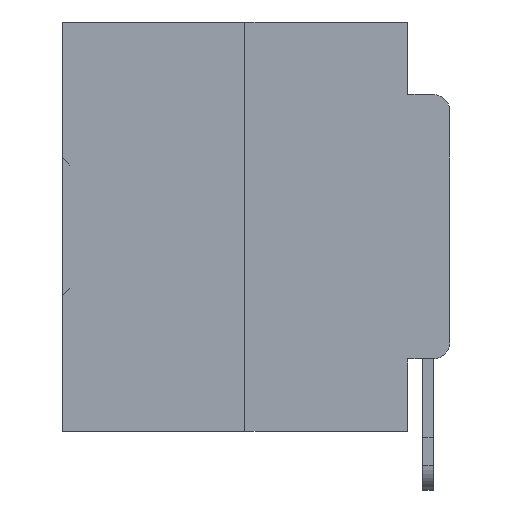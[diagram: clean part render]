
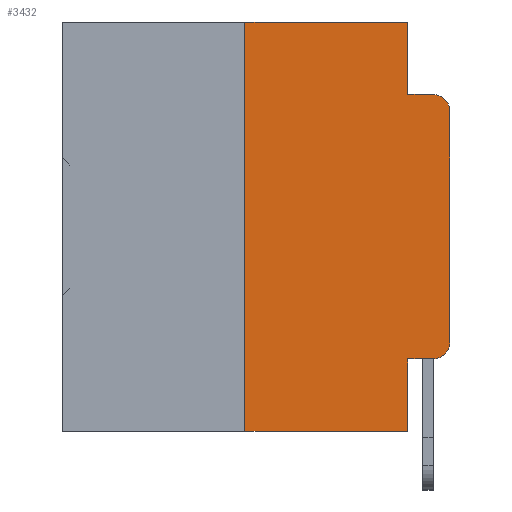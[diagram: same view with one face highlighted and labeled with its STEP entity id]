
A CAD part, left-side view. The second image highlights one B-rep face of the part: STEP entity #3432.
In plain terms, the highlighted planar face has unit normal (-1, 0, 0).
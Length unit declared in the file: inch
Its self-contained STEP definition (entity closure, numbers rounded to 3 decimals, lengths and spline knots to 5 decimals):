
#521 = CARTESIAN_POINT ( 'NONE',  ( 0., 0.051, 0. ) ) ;
#569 = ORIENTED_EDGE ( 'NONE', *, *, #15736, .F. ) ;
#796 = VERTEX_POINT ( 'NONE', #5064 ) ;
#1227 = AXIS2_PLACEMENT_3D ( 'NONE', #4578, #33286, #16240 ) ;
#1296 = LINE ( 'NONE', #9260, #24424 ) ;
#2381 = ORIENTED_EDGE ( 'NONE', *, *, #10385, .T. ) ;
#2824 = VERTEX_POINT ( 'NONE', #27912 ) ;
#3432 = ADVANCED_FACE ( 'NONE', ( #32026 ), #13375, .F. ) ;
#3728 = LINE ( 'NONE', #521, #25884 ) ;
#3797 = ORIENTED_EDGE ( 'NONE', *, *, #16546, .F. ) ;
#4196 = DIRECTION ( 'NONE',  ( -1., 0., 0. ) ) ;
#4578 = CARTESIAN_POINT ( 'NONE',  ( 0., 0.473, 0. ) ) ;
#4650 = VERTEX_POINT ( 'NONE', #30499 ) ;
#5064 = CARTESIAN_POINT ( 'NONE',  ( 0., 0.25, 0. ) ) ;
#5159 = DIRECTION ( 'NONE',  ( 0., -1., 0. ) ) ;
#8352 = CARTESIAN_POINT ( 'NONE',  ( 0., 0.051, -0.0885 ) ) ;
#9185 = CARTESIAN_POINT ( 'NONE',  ( 0., 0., 0. ) ) ;
#9260 = CARTESIAN_POINT ( 'NONE',  ( 0., 0.25, 0. ) ) ;
#9887 = CIRCLE ( 'NONE', #21620, 0.02 ) ;
#10050 = EDGE_CURVE ( 'NONE', #2824, #24949, #9887, .T. ) ;
#10385 = EDGE_CURVE ( 'NONE', #24949, #16553, #22860, .T. ) ;
#10541 = CARTESIAN_POINT ( 'NONE',  ( 0., 0.051, -0.4115 ) ) ;
#11110 = CARTESIAN_POINT ( 'NONE',  ( 0., 0.051, 0. ) ) ;
#11295 = CARTESIAN_POINT ( 'NONE',  ( 0., 0.02, -0.1085 ) ) ;
#11695 = VERTEX_POINT ( 'NONE', #31929 ) ;
#11756 = EDGE_CURVE ( 'NONE', #17212, #4650, #3728, .T. ) ;
#12059 = DIRECTION ( 'NONE',  ( 0., 0., 1. ) ) ;
#12269 = LINE ( 'NONE', #17096, #34062 ) ;
#12294 = VECTOR ( 'NONE', #15080, 39.37008 ) ;
#12542 = ORIENTED_EDGE ( 'NONE', *, *, #14366, .T. ) ;
#12704 = CARTESIAN_POINT ( 'NONE',  ( 0., 0.051, -0.4115 ) ) ;
#12941 = EDGE_CURVE ( 'NONE', #11695, #796, #1296, .T. ) ;
#13375 = PLANE ( 'NONE',  #1227 ) ;
#13400 = ORIENTED_EDGE ( 'NONE', *, *, #19215, .F. ) ;
#13410 = DIRECTION ( 'NONE',  ( 0., -1., 0. ) ) ;
#14172 = DIRECTION ( 'NONE',  ( 0., 0., -1. ) ) ;
#14339 = DIRECTION ( 'NONE',  ( 0., -1., 0. ) ) ;
#14366 = EDGE_CURVE ( 'NONE', #17212, #2824, #23457, .T. ) ;
#15010 = CARTESIAN_POINT ( 'NONE',  ( 0., 0., -0.1085 ) ) ;
#15080 = DIRECTION ( 'NONE',  ( 0., 0., -1. ) ) ;
#15127 = CARTESIAN_POINT ( 'NONE',  ( 0., 0., -0.3915 ) ) ;
#15662 = VERTEX_POINT ( 'NONE', #30761 ) ;
#15736 = EDGE_CURVE ( 'NONE', #796, #33041, #18391, .T. ) ;
#16240 = DIRECTION ( 'NONE',  ( 0., 0., -1. ) ) ;
#16546 = EDGE_CURVE ( 'NONE', #26595, #15662, #27702, .T. ) ;
#16553 = VERTEX_POINT ( 'NONE', #15010 ) ;
#16678 = CARTESIAN_POINT ( 'NONE',  ( 0., 0.473, 0. ) ) ;
#17096 = CARTESIAN_POINT ( 'NONE',  ( 0., 0.473, -0.5 ) ) ;
#17212 = VERTEX_POINT ( 'NONE', #12704 ) ;
#17490 = VECTOR ( 'NONE', #5159, 39.37008 ) ;
#18391 = LINE ( 'NONE', #16678, #17490 ) ;
#19215 = EDGE_CURVE ( 'NONE', #33041, #26595, #33208, .T. ) ;
#19676 = ORIENTED_EDGE ( 'NONE', *, *, #30420, .T. ) ;
#21546 = CARTESIAN_POINT ( 'NONE',  ( 0., 0.02, -0.3915 ) ) ;
#21620 = AXIS2_PLACEMENT_3D ( 'NONE', #21546, #4196, #24394 ) ;
#22612 = CIRCLE ( 'NONE', #31971, 0.02 ) ;
#22860 = LINE ( 'NONE', #9185, #27752 ) ;
#23457 = LINE ( 'NONE', #10541, #28319 ) ;
#24174 = ORIENTED_EDGE ( 'NONE', *, *, #27209, .T. ) ;
#24394 = DIRECTION ( 'NONE',  ( 0., 0., -1. ) ) ;
#24424 = VECTOR ( 'NONE', #29253, 39.37008 ) ;
#24949 = VERTEX_POINT ( 'NONE', #15127 ) ;
#25199 = EDGE_LOOP ( 'NONE', ( #2381, #19676, #3797, #13400, #569, #29070, #24174, #33466, #12542, #27751 ) ) ;
#25884 = VECTOR ( 'NONE', #26496, 39.37008 ) ;
#26399 = DIRECTION ( 'NONE',  ( 0., -1., 0. ) ) ;
#26496 = DIRECTION ( 'NONE',  ( 0., 0., -1. ) ) ;
#26595 = VERTEX_POINT ( 'NONE', #8352 ) ;
#27209 = EDGE_CURVE ( 'NONE', #11695, #4650, #12269, .T. ) ;
#27702 = LINE ( 'NONE', #29114, #35175 ) ;
#27751 = ORIENTED_EDGE ( 'NONE', *, *, #10050, .T. ) ;
#27752 = VECTOR ( 'NONE', #12059, 39.37008 ) ;
#27912 = CARTESIAN_POINT ( 'NONE',  ( 0., 0.02, -0.4115 ) ) ;
#28319 = VECTOR ( 'NONE', #13410, 39.37008 ) ;
#29070 = ORIENTED_EDGE ( 'NONE', *, *, #12941, .F. ) ;
#29114 = CARTESIAN_POINT ( 'NONE',  ( 0., 0.051, -0.0885 ) ) ;
#29253 = DIRECTION ( 'NONE',  ( 0., 0., 1. ) ) ;
#29329 = CARTESIAN_POINT ( 'NONE',  ( 0., 0.051, 0. ) ) ;
#30420 = EDGE_CURVE ( 'NONE', #16553, #15662, #22612, .T. ) ;
#30499 = CARTESIAN_POINT ( 'NONE',  ( 0., 0.051, -0.5 ) ) ;
#30761 = CARTESIAN_POINT ( 'NONE',  ( 0., 0.02, -0.0885 ) ) ;
#31222 = DIRECTION ( 'NONE',  ( -1., 0., 0. ) ) ;
#31929 = CARTESIAN_POINT ( 'NONE',  ( 0., 0.25, -0.5 ) ) ;
#31971 = AXIS2_PLACEMENT_3D ( 'NONE', #11295, #31222, #14172 ) ;
#32026 = FACE_OUTER_BOUND ( 'NONE', #25199, .T. ) ;
#33041 = VERTEX_POINT ( 'NONE', #11110 ) ;
#33208 = LINE ( 'NONE', #29329, #12294 ) ;
#33286 = DIRECTION ( 'NONE',  ( 1., 0., 0. ) ) ;
#33466 = ORIENTED_EDGE ( 'NONE', *, *, #11756, .F. ) ;
#34062 = VECTOR ( 'NONE', #14339, 39.37008 ) ;
#35175 = VECTOR ( 'NONE', #26399, 39.37008 ) ;
